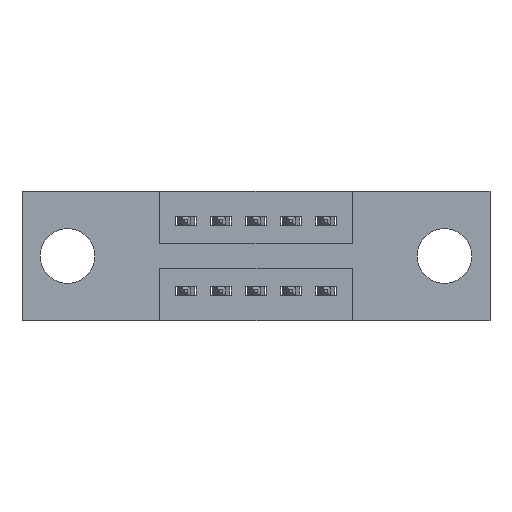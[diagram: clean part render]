
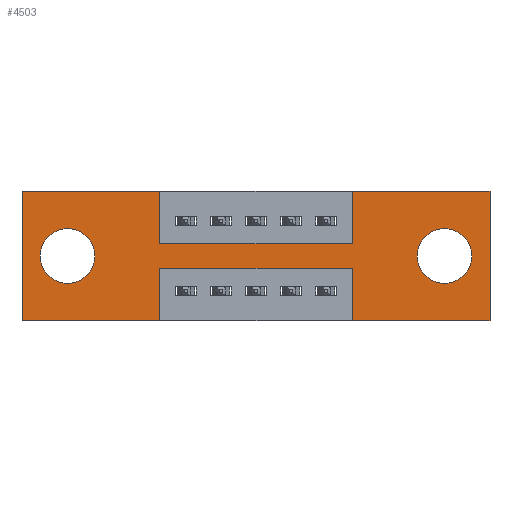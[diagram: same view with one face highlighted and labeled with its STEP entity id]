
A CAD part, front view. The second image highlights one B-rep face of the part: STEP entity #4503.
In plain terms, the highlighted planar face has unit normal (0, -1, 0).
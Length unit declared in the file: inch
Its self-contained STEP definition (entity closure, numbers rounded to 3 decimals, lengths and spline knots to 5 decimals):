
#90 = DIRECTION ( 'NONE',  ( 0., 1., 0. ) ) ;
#92 = DIRECTION ( 'NONE',  ( 1., 0., 0. ) ) ;
#160 = CARTESIAN_POINT ( 'NONE',  ( 0., 0., 0. ) ) ;
#202 = EDGE_CURVE ( 'NONE', #5466, #2025, #5014, .T. ) ;
#266 = EDGE_CURVE ( 'NONE', #8878, #4226, #8101, .T. ) ;
#350 = ORIENTED_EDGE ( 'NONE', *, *, #1061, .F. ) ;
#359 = EDGE_CURVE ( 'NONE', #530, #5961, #3803, .T. ) ;
#376 = VERTEX_POINT ( 'NONE', #5408 ) ;
#412 = CARTESIAN_POINT ( 'NONE',  ( 1.335, 0., 0. ) ) ;
#463 = CARTESIAN_POINT ( 'NONE',  ( 1.205, 0., -0.185 ) ) ;
#471 = DIRECTION ( 'NONE',  ( -1., 0., 0. ) ) ;
#501 = LINE ( 'NONE', #160, #7770 ) ;
#530 = VERTEX_POINT ( 'NONE', #1866 ) ;
#611 = CARTESIAN_POINT ( 'NONE',  ( 0., 0., 0. ) ) ;
#690 = VECTOR ( 'NONE', #6342, 39.37008 ) ;
#783 = ORIENTED_EDGE ( 'NONE', *, *, #3022, .F. ) ;
#798 = LINE ( 'NONE', #6395, #6090 ) ;
#826 = CIRCLE ( 'NONE', #1997, 0.078 ) ;
#902 = LINE ( 'NONE', #8141, #8065 ) ;
#1048 = DIRECTION ( 'NONE',  ( 0., 0., 1. ) ) ;
#1061 = EDGE_CURVE ( 'NONE', #1294, #8256, #7895, .T. ) ;
#1091 = AXIS2_PLACEMENT_3D ( 'NONE', #3085, #5804, #2661 ) ;
#1294 = VERTEX_POINT ( 'NONE', #412 ) ;
#1355 = DIRECTION ( 'NONE',  ( 0., 0., -1. ) ) ;
#1390 = LINE ( 'NONE', #6580, #6821 ) ;
#1484 = EDGE_CURVE ( 'NONE', #8188, #1653, #798, .T. ) ;
#1586 = FACE_BOUND ( 'NONE', #3481, .T. ) ;
#1653 = VERTEX_POINT ( 'NONE', #4932 ) ;
#1672 = VECTOR ( 'NONE', #7325, 39.37008 ) ;
#1754 = EDGE_LOOP ( 'NONE', ( #8551, #4948, #2082, #8652, #350, #783, #7721, #1900, #8274, #7591, #7511, #3046 ) ) ;
#1858 = EDGE_CURVE ( 'NONE', #7415, #6685, #7308, .T. ) ;
#1866 = CARTESIAN_POINT ( 'NONE',  ( 0.13, 0., -0.263 ) ) ;
#1871 = EDGE_CURVE ( 'NONE', #4226, #3556, #5555, .T. ) ;
#1900 = ORIENTED_EDGE ( 'NONE', *, *, #5373, .F. ) ;
#1907 = DIRECTION ( 'NONE',  ( 0., 0., 1. ) ) ;
#1997 = AXIS2_PLACEMENT_3D ( 'NONE', #2866, #7659, #3504 ) ;
#2025 = VERTEX_POINT ( 'NONE', #2581 ) ;
#2082 = ORIENTED_EDGE ( 'NONE', *, *, #1484, .F. ) ;
#2194 = AXIS2_PLACEMENT_3D ( 'NONE', #463, #90, #1355 ) ;
#2297 = FACE_OUTER_BOUND ( 'NONE', #1754, .T. ) ;
#2506 = CARTESIAN_POINT ( 'NONE',  ( 0.13, 0., -0.185 ) ) ;
#2508 = DIRECTION ( 'NONE',  ( -1., 0., 0. ) ) ;
#2581 = CARTESIAN_POINT ( 'NONE',  ( 1.205, 0., -0.107 ) ) ;
#2621 = CARTESIAN_POINT ( 'NONE',  ( 0., 0., -0.37 ) ) ;
#2661 = DIRECTION ( 'NONE',  ( 0., 0., -1. ) ) ;
#2680 = PLANE ( 'NONE',  #1091 ) ;
#2695 = CIRCLE ( 'NONE', #7827, 0.078 ) ;
#2866 = CARTESIAN_POINT ( 'NONE',  ( 1.205, 0., -0.185 ) ) ;
#2883 = CARTESIAN_POINT ( 'NONE',  ( 0., 0., 0. ) ) ;
#3007 = EDGE_LOOP ( 'NONE', ( #8938, #8394 ) ) ;
#3022 = EDGE_CURVE ( 'NONE', #376, #1294, #1390, .T. ) ;
#3046 = ORIENTED_EDGE ( 'NONE', *, *, #266, .F. ) ;
#3085 = CARTESIAN_POINT ( 'NONE',  ( 0., 0., -0.37 ) ) ;
#3154 = EDGE_CURVE ( 'NONE', #5961, #530, #2695, .T. ) ;
#3178 = CARTESIAN_POINT ( 'NONE',  ( 0.9425, 0., 0. ) ) ;
#3227 = VECTOR ( 'NONE', #8294, 39.37008 ) ;
#3342 = VERTEX_POINT ( 'NONE', #7552 ) ;
#3434 = LINE ( 'NONE', #8202, #3227 ) ;
#3454 = CARTESIAN_POINT ( 'NONE',  ( 1.335, 0., -0.37 ) ) ;
#3481 = EDGE_LOOP ( 'NONE', ( #8466, #8610 ) ) ;
#3504 = DIRECTION ( 'NONE',  ( 0., 0., -1. ) ) ;
#3545 = AXIS2_PLACEMENT_3D ( 'NONE', #6005, #5998, #5985 ) ;
#3556 = VERTEX_POINT ( 'NONE', #611 ) ;
#3574 = VECTOR ( 'NONE', #1907, 39.37008 ) ;
#3665 = EDGE_CURVE ( 'NONE', #8256, #8188, #902, .T. ) ;
#3739 = LINE ( 'NONE', #8718, #5513 ) ;
#3775 = VECTOR ( 'NONE', #4578, 39.37008 ) ;
#3803 = CIRCLE ( 'NONE', #3545, 0.078 ) ;
#4053 = VERTEX_POINT ( 'NONE', #5602 ) ;
#4226 = VERTEX_POINT ( 'NONE', #8380 ) ;
#4258 = CARTESIAN_POINT ( 'NONE',  ( 0.3925, 0., 0. ) ) ;
#4503 = ADVANCED_FACE ( 'NONE', ( #5411, #1586, #2297 ), #2680, .T. ) ;
#4578 = DIRECTION ( 'NONE',  ( 0., 0., -1. ) ) ;
#4868 = CARTESIAN_POINT ( 'NONE',  ( 0.9425, 0., -0.37 ) ) ;
#4932 = CARTESIAN_POINT ( 'NONE',  ( 0.9425, 0., -0.22 ) ) ;
#4948 = ORIENTED_EDGE ( 'NONE', *, *, #8132, .F. ) ;
#5014 = CIRCLE ( 'NONE', #2194, 0.078 ) ;
#5032 = EDGE_CURVE ( 'NONE', #3342, #8878, #3434, .T. ) ;
#5352 = CARTESIAN_POINT ( 'NONE',  ( 0.3925, 0., -0.37 ) ) ;
#5373 = EDGE_CURVE ( 'NONE', #6685, #4053, #6555, .T. ) ;
#5408 = CARTESIAN_POINT ( 'NONE',  ( 0.9425, 0., 0. ) ) ;
#5411 = FACE_BOUND ( 'NONE', #3007, .T. ) ;
#5466 = VERTEX_POINT ( 'NONE', #5883 ) ;
#5513 = VECTOR ( 'NONE', #471, 39.37008 ) ;
#5555 = LINE ( 'NONE', #2883, #3574 ) ;
#5572 = EDGE_CURVE ( 'NONE', #4053, #376, #6859, .T. ) ;
#5602 = CARTESIAN_POINT ( 'NONE',  ( 0.9425, 0., -0.15 ) ) ;
#5804 = DIRECTION ( 'NONE',  ( 0., -1., 0. ) ) ;
#5858 = EDGE_CURVE ( 'NONE', #2025, #5466, #826, .T. ) ;
#5883 = CARTESIAN_POINT ( 'NONE',  ( 1.205, 0., -0.263 ) ) ;
#5961 = VERTEX_POINT ( 'NONE', #7106 ) ;
#5985 = DIRECTION ( 'NONE',  ( 0., 0., 1. ) ) ;
#5998 = DIRECTION ( 'NONE',  ( 0., 1., 0. ) ) ;
#6005 = CARTESIAN_POINT ( 'NONE',  ( 0.13, 0., -0.185 ) ) ;
#6090 = VECTOR ( 'NONE', #7817, 39.37008 ) ;
#6201 = VECTOR ( 'NONE', #8588, 39.37008 ) ;
#6342 = DIRECTION ( 'NONE',  ( -1., 0., 0. ) ) ;
#6395 = CARTESIAN_POINT ( 'NONE',  ( 0.9425, 0., -0.37 ) ) ;
#6531 = CARTESIAN_POINT ( 'NONE',  ( 0.3925, 0., 0. ) ) ;
#6551 = DIRECTION ( 'NONE',  ( 1., 0., 0. ) ) ;
#6555 = LINE ( 'NONE', #8838, #8196 ) ;
#6580 = CARTESIAN_POINT ( 'NONE',  ( 0., 0., 0. ) ) ;
#6685 = VERTEX_POINT ( 'NONE', #7152 ) ;
#6821 = VECTOR ( 'NONE', #6551, 39.37008 ) ;
#6859 = LINE ( 'NONE', #3178, #1672 ) ;
#7106 = CARTESIAN_POINT ( 'NONE',  ( 0.13, 0., -0.107 ) ) ;
#7152 = CARTESIAN_POINT ( 'NONE',  ( 0.3925, 0., -0.15 ) ) ;
#7308 = LINE ( 'NONE', #6531, #3775 ) ;
#7325 = DIRECTION ( 'NONE',  ( 0., 0., 1. ) ) ;
#7415 = VERTEX_POINT ( 'NONE', #4258 ) ;
#7511 = ORIENTED_EDGE ( 'NONE', *, *, #1871, .F. ) ;
#7552 = CARTESIAN_POINT ( 'NONE',  ( 0.3925, 0., -0.22 ) ) ;
#7591 = ORIENTED_EDGE ( 'NONE', *, *, #7683, .F. ) ;
#7659 = DIRECTION ( 'NONE',  ( 0., 1., 0. ) ) ;
#7683 = EDGE_CURVE ( 'NONE', #3556, #7415, #501, .T. ) ;
#7721 = ORIENTED_EDGE ( 'NONE', *, *, #5572, .F. ) ;
#7770 = VECTOR ( 'NONE', #7923, 39.37008 ) ;
#7817 = DIRECTION ( 'NONE',  ( 0., 0., 1. ) ) ;
#7827 = AXIS2_PLACEMENT_3D ( 'NONE', #2506, #8782, #1048 ) ;
#7895 = LINE ( 'NONE', #8684, #6201 ) ;
#7923 = DIRECTION ( 'NONE',  ( 1., 0., 0. ) ) ;
#8065 = VECTOR ( 'NONE', #2508, 39.37008 ) ;
#8101 = LINE ( 'NONE', #2621, #690 ) ;
#8132 = EDGE_CURVE ( 'NONE', #1653, #3342, #3739, .T. ) ;
#8141 = CARTESIAN_POINT ( 'NONE',  ( 0., 0., -0.37 ) ) ;
#8188 = VERTEX_POINT ( 'NONE', #4868 ) ;
#8196 = VECTOR ( 'NONE', #92, 39.37008 ) ;
#8202 = CARTESIAN_POINT ( 'NONE',  ( 0.3925, 0., -0.37 ) ) ;
#8256 = VERTEX_POINT ( 'NONE', #3454 ) ;
#8274 = ORIENTED_EDGE ( 'NONE', *, *, #1858, .F. ) ;
#8294 = DIRECTION ( 'NONE',  ( 0., 0., -1. ) ) ;
#8380 = CARTESIAN_POINT ( 'NONE',  ( 0., 0., -0.37 ) ) ;
#8394 = ORIENTED_EDGE ( 'NONE', *, *, #202, .T. ) ;
#8466 = ORIENTED_EDGE ( 'NONE', *, *, #3154, .T. ) ;
#8551 = ORIENTED_EDGE ( 'NONE', *, *, #5032, .F. ) ;
#8588 = DIRECTION ( 'NONE',  ( 0., 0., -1. ) ) ;
#8610 = ORIENTED_EDGE ( 'NONE', *, *, #359, .T. ) ;
#8652 = ORIENTED_EDGE ( 'NONE', *, *, #3665, .F. ) ;
#8684 = CARTESIAN_POINT ( 'NONE',  ( 1.335, 0., 0. ) ) ;
#8718 = CARTESIAN_POINT ( 'NONE',  ( 0.3925, 0., -0.22 ) ) ;
#8782 = DIRECTION ( 'NONE',  ( 0., 1., 0. ) ) ;
#8838 = CARTESIAN_POINT ( 'NONE',  ( 0.3925, 0., -0.15 ) ) ;
#8878 = VERTEX_POINT ( 'NONE', #5352 ) ;
#8938 = ORIENTED_EDGE ( 'NONE', *, *, #5858, .T. ) ;
